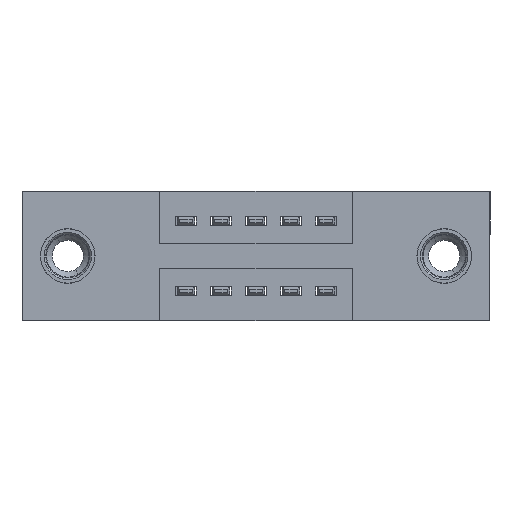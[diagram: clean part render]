
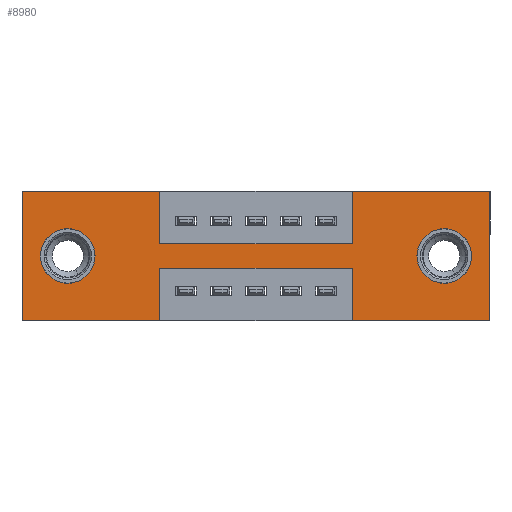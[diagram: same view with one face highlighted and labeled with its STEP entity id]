
A CAD part, front view. The second image highlights one B-rep face of the part: STEP entity #8980.
In plain terms, the highlighted planar face has unit normal (0, -1, 0).
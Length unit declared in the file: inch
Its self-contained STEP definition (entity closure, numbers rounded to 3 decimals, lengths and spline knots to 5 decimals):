
#19 = CARTESIAN_POINT ( 'NONE',  ( 0.9425, 0., -0.15 ) ) ;
#128 = CARTESIAN_POINT ( 'NONE',  ( 0., 0., 0. ) ) ;
#152 = CIRCLE ( 'NONE', #13033, 0.078 ) ;
#179 = EDGE_LOOP ( 'NONE', ( #3639, #10919 ) ) ;
#259 = VECTOR ( 'NONE', #2491, 39.37008 ) ;
#301 = CARTESIAN_POINT ( 'NONE',  ( 0.3925, 0., 0. ) ) ;
#312 = EDGE_LOOP ( 'NONE', ( #6293, #2550, #10890, #4994, #2939, #12785, #1828, #12977, #5636, #6755, #11566, #6358 ) ) ;
#387 = VECTOR ( 'NONE', #11338, 39.37008 ) ;
#521 = VECTOR ( 'NONE', #8468, 39.37008 ) ;
#544 = LINE ( 'NONE', #8040, #387 ) ;
#614 = CARTESIAN_POINT ( 'NONE',  ( 0.13, 0., -0.185 ) ) ;
#633 = FACE_BOUND ( 'NONE', #6962, .T. ) ;
#890 = DIRECTION ( 'NONE',  ( 0., 1., 0. ) ) ;
#975 = FACE_OUTER_BOUND ( 'NONE', #312, .T. ) ;
#1540 = CARTESIAN_POINT ( 'NONE',  ( 0., 0., -0.37 ) ) ;
#1584 = VECTOR ( 'NONE', #12752, 39.37008 ) ;
#1611 = EDGE_CURVE ( 'NONE', #3738, #10755, #6556, .T. ) ;
#1625 = CARTESIAN_POINT ( 'NONE',  ( 1.335, 0., -0.37 ) ) ;
#1668 = VERTEX_POINT ( 'NONE', #12847 ) ;
#1719 = CARTESIAN_POINT ( 'NONE',  ( 0.13, 0., -0.107 ) ) ;
#1828 = ORIENTED_EDGE ( 'NONE', *, *, #10768, .F. ) ;
#1989 = DIRECTION ( 'NONE',  ( 0., 0., -1. ) ) ;
#2303 = EDGE_CURVE ( 'NONE', #6918, #2342, #152, .T. ) ;
#2342 = VERTEX_POINT ( 'NONE', #1719 ) ;
#2393 = VERTEX_POINT ( 'NONE', #7077 ) ;
#2424 = LINE ( 'NONE', #5354, #12848 ) ;
#2487 = LINE ( 'NONE', #8666, #3944 ) ;
#2491 = DIRECTION ( 'NONE',  ( 0., 0., 1. ) ) ;
#2524 = VECTOR ( 'NONE', #10188, 39.37008 ) ;
#2550 = ORIENTED_EDGE ( 'NONE', *, *, #4261, .F. ) ;
#2890 = CARTESIAN_POINT ( 'NONE',  ( 0.13, 0., -0.185 ) ) ;
#2939 = ORIENTED_EDGE ( 'NONE', *, *, #11975, .F. ) ;
#3236 = LINE ( 'NONE', #301, #4228 ) ;
#3504 = CARTESIAN_POINT ( 'NONE',  ( 1.205, 0., -0.185 ) ) ;
#3621 = CARTESIAN_POINT ( 'NONE',  ( 1.205, 0., -0.263 ) ) ;
#3629 = VERTEX_POINT ( 'NONE', #9642 ) ;
#3639 = ORIENTED_EDGE ( 'NONE', *, *, #1611, .T. ) ;
#3654 = LINE ( 'NONE', #9939, #11664 ) ;
#3704 = VERTEX_POINT ( 'NONE', #5666 ) ;
#3738 = VERTEX_POINT ( 'NONE', #6674 ) ;
#3781 = AXIS2_PLACEMENT_3D ( 'NONE', #3504, #7653, #7737 ) ;
#3840 = VERTEX_POINT ( 'NONE', #1625 ) ;
#3944 = VECTOR ( 'NONE', #8754, 39.37008 ) ;
#4110 = DIRECTION ( 'NONE',  ( 0., 0., 1. ) ) ;
#4228 = VECTOR ( 'NONE', #7592, 39.37008 ) ;
#4261 = EDGE_CURVE ( 'NONE', #3629, #2393, #4360, .T. ) ;
#4285 = VECTOR ( 'NONE', #9375, 39.37008 ) ;
#4360 = LINE ( 'NONE', #10644, #1584 ) ;
#4994 = ORIENTED_EDGE ( 'NONE', *, *, #6812, .F. ) ;
#5183 = VECTOR ( 'NONE', #5255, 39.37008 ) ;
#5255 = DIRECTION ( 'NONE',  ( -1., 0., 0. ) ) ;
#5354 = CARTESIAN_POINT ( 'NONE',  ( 0.3925, 0., -0.15 ) ) ;
#5400 = DIRECTION ( 'NONE',  ( 1., 0., 0. ) ) ;
#5423 = EDGE_CURVE ( 'NONE', #10902, #9805, #5612, .T. ) ;
#5460 = EDGE_CURVE ( 'NONE', #10755, #3738, #6090, .T. ) ;
#5516 = CARTESIAN_POINT ( 'NONE',  ( 1.335, 0., 0. ) ) ;
#5535 = FACE_BOUND ( 'NONE', #179, .T. ) ;
#5612 = LINE ( 'NONE', #8028, #2524 ) ;
#5636 = ORIENTED_EDGE ( 'NONE', *, *, #8895, .F. ) ;
#5666 = CARTESIAN_POINT ( 'NONE',  ( 0.9425, 0., -0.37 ) ) ;
#5738 = EDGE_CURVE ( 'NONE', #3704, #3629, #12462, .T. ) ;
#5995 = DIRECTION ( 'NONE',  ( 0., 1., 0. ) ) ;
#6090 = CIRCLE ( 'NONE', #12730, 0.078 ) ;
#6225 = LINE ( 'NONE', #128, #521 ) ;
#6293 = ORIENTED_EDGE ( 'NONE', *, *, #6889, .F. ) ;
#6358 = ORIENTED_EDGE ( 'NONE', *, *, #9223, .F. ) ;
#6401 = CARTESIAN_POINT ( 'NONE',  ( 0., 0., -0.37 ) ) ;
#6546 = VERTEX_POINT ( 'NONE', #10274 ) ;
#6556 = CIRCLE ( 'NONE', #3781, 0.078 ) ;
#6674 = CARTESIAN_POINT ( 'NONE',  ( 1.205, 0., -0.107 ) ) ;
#6742 = AXIS2_PLACEMENT_3D ( 'NONE', #2890, #5995, #13282 ) ;
#6755 = ORIENTED_EDGE ( 'NONE', *, *, #5423, .F. ) ;
#6812 = EDGE_CURVE ( 'NONE', #3840, #3704, #10325, .T. ) ;
#6817 = VERTEX_POINT ( 'NONE', #19 ) ;
#6889 = EDGE_CURVE ( 'NONE', #2393, #6546, #2487, .T. ) ;
#6918 = VERTEX_POINT ( 'NONE', #12895 ) ;
#6962 = EDGE_LOOP ( 'NONE', ( #8253, #7053 ) ) ;
#7053 = ORIENTED_EDGE ( 'NONE', *, *, #2303, .T. ) ;
#7077 = CARTESIAN_POINT ( 'NONE',  ( 0.3925, 0., -0.22 ) ) ;
#7290 = VERTEX_POINT ( 'NONE', #11346 ) ;
#7592 = DIRECTION ( 'NONE',  ( 0., 0., -1. ) ) ;
#7653 = DIRECTION ( 'NONE',  ( 0., 1., 0. ) ) ;
#7737 = DIRECTION ( 'NONE',  ( 0., 0., -1. ) ) ;
#7932 = CARTESIAN_POINT ( 'NONE',  ( 0., 0., 0. ) ) ;
#8028 = CARTESIAN_POINT ( 'NONE',  ( 0., 0., 0. ) ) ;
#8040 = CARTESIAN_POINT ( 'NONE',  ( 0., 0., 0. ) ) ;
#8089 = LINE ( 'NONE', #8858, #259 ) ;
#8220 = CARTESIAN_POINT ( 'NONE',  ( 1.205, 0., -0.185 ) ) ;
#8253 = ORIENTED_EDGE ( 'NONE', *, *, #10442, .T. ) ;
#8468 = DIRECTION ( 'NONE',  ( 0., 0., 1. ) ) ;
#8666 = CARTESIAN_POINT ( 'NONE',  ( 0.3925, 0., -0.37 ) ) ;
#8754 = DIRECTION ( 'NONE',  ( 0., 0., -1. ) ) ;
#8858 = CARTESIAN_POINT ( 'NONE',  ( 0.9425, 0., 0. ) ) ;
#8860 = DIRECTION ( 'NONE',  ( 0., 0., -1. ) ) ;
#8895 = EDGE_CURVE ( 'NONE', #9805, #1668, #3236, .T. ) ;
#8939 = LINE ( 'NONE', #6401, #5183 ) ;
#8980 = ADVANCED_FACE ( 'NONE', ( #5535, #633, #975 ), #12958, .T. ) ;
#9201 = EDGE_CURVE ( 'NONE', #1668, #6817, #2424, .T. ) ;
#9223 = EDGE_CURVE ( 'NONE', #6546, #11803, #8939, .T. ) ;
#9254 = CIRCLE ( 'NONE', #6742, 0.078 ) ;
#9305 = CARTESIAN_POINT ( 'NONE',  ( 0.9425, 0., -0.37 ) ) ;
#9375 = DIRECTION ( 'NONE',  ( -1., 0., 0. ) ) ;
#9642 = CARTESIAN_POINT ( 'NONE',  ( 0.9425, 0., -0.22 ) ) ;
#9692 = VECTOR ( 'NONE', #4110, 39.37008 ) ;
#9805 = VERTEX_POINT ( 'NONE', #10036 ) ;
#9939 = CARTESIAN_POINT ( 'NONE',  ( 1.335, 0., 0. ) ) ;
#9977 = DIRECTION ( 'NONE',  ( 0., 0., 1. ) ) ;
#10036 = CARTESIAN_POINT ( 'NONE',  ( 0.3925, 0., 0. ) ) ;
#10188 = DIRECTION ( 'NONE',  ( 1., 0., 0. ) ) ;
#10274 = CARTESIAN_POINT ( 'NONE',  ( 0.3925, 0., -0.37 ) ) ;
#10325 = LINE ( 'NONE', #10621, #4285 ) ;
#10442 = EDGE_CURVE ( 'NONE', #2342, #6918, #9254, .T. ) ;
#10621 = CARTESIAN_POINT ( 'NONE',  ( 0., 0., -0.37 ) ) ;
#10644 = CARTESIAN_POINT ( 'NONE',  ( 0.3925, 0., -0.22 ) ) ;
#10755 = VERTEX_POINT ( 'NONE', #3621 ) ;
#10768 = EDGE_CURVE ( 'NONE', #6817, #7290, #8089, .T. ) ;
#10890 = ORIENTED_EDGE ( 'NONE', *, *, #5738, .F. ) ;
#10902 = VERTEX_POINT ( 'NONE', #7932 ) ;
#10919 = ORIENTED_EDGE ( 'NONE', *, *, #5460, .T. ) ;
#11124 = DIRECTION ( 'NONE',  ( 0., 0., -1. ) ) ;
#11283 = AXIS2_PLACEMENT_3D ( 'NONE', #1540, #11941, #8860 ) ;
#11338 = DIRECTION ( 'NONE',  ( 1., 0., 0. ) ) ;
#11346 = CARTESIAN_POINT ( 'NONE',  ( 0.9425, 0., 0. ) ) ;
#11566 = ORIENTED_EDGE ( 'NONE', *, *, #13383, .F. ) ;
#11664 = VECTOR ( 'NONE', #11124, 39.37008 ) ;
#11803 = VERTEX_POINT ( 'NONE', #12792 ) ;
#11839 = VERTEX_POINT ( 'NONE', #5516 ) ;
#11941 = DIRECTION ( 'NONE',  ( 0., -1., 0. ) ) ;
#11975 = EDGE_CURVE ( 'NONE', #11839, #3840, #3654, .T. ) ;
#12093 = EDGE_CURVE ( 'NONE', #7290, #11839, #544, .T. ) ;
#12462 = LINE ( 'NONE', #9305, #9692 ) ;
#12730 = AXIS2_PLACEMENT_3D ( 'NONE', #8220, #890, #1989 ) ;
#12752 = DIRECTION ( 'NONE',  ( -1., 0., 0. ) ) ;
#12785 = ORIENTED_EDGE ( 'NONE', *, *, #12093, .F. ) ;
#12792 = CARTESIAN_POINT ( 'NONE',  ( 0., 0., -0.37 ) ) ;
#12847 = CARTESIAN_POINT ( 'NONE',  ( 0.3925, 0., -0.15 ) ) ;
#12848 = VECTOR ( 'NONE', #5400, 39.37008 ) ;
#12895 = CARTESIAN_POINT ( 'NONE',  ( 0.13, 0., -0.263 ) ) ;
#12958 = PLANE ( 'NONE',  #11283 ) ;
#12977 = ORIENTED_EDGE ( 'NONE', *, *, #9201, .F. ) ;
#13033 = AXIS2_PLACEMENT_3D ( 'NONE', #614, #13270, #9977 ) ;
#13270 = DIRECTION ( 'NONE',  ( 0., 1., 0. ) ) ;
#13282 = DIRECTION ( 'NONE',  ( 0., 0., 1. ) ) ;
#13383 = EDGE_CURVE ( 'NONE', #11803, #10902, #6225, .T. ) ;
